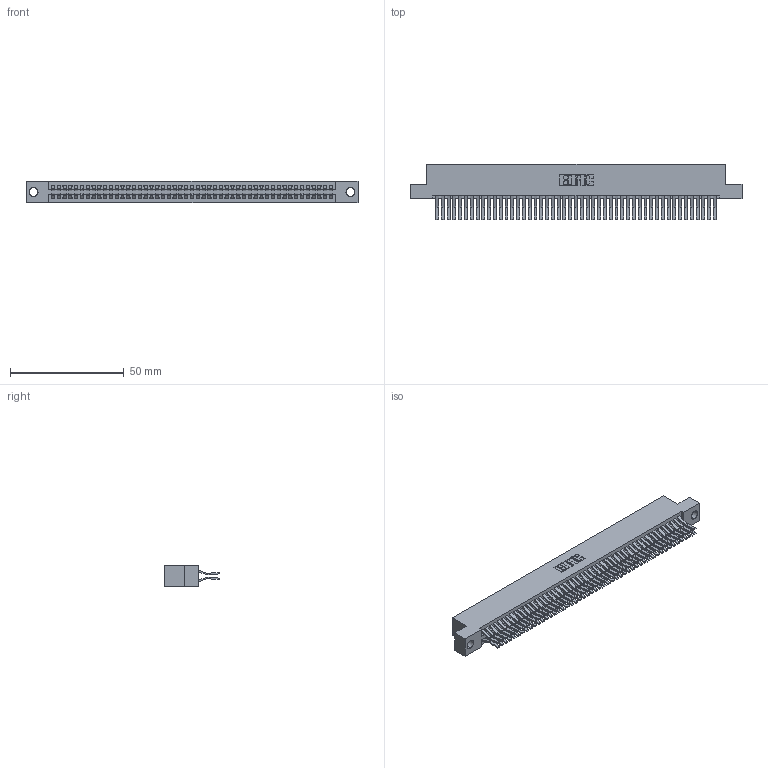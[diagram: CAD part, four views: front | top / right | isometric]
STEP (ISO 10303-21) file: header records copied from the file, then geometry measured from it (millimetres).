
FILE_DESCRIPTION (( 'STEP AP203' ), '1' );
FILE_NAME ('345-098-560-204.STEP', '2021-05-20T18:23:55', ( '' ), ( '' ), 'SwSTEP 2.0', 'SolidWorks 2020', '' );
FILE_SCHEMA (( 'CONFIG_CONTROL_DESIGN' ));
Length unit declared in the file: inch
Products named in the file (3): 345 Part_Flush Mounting Lugs - 0.156 Dia-TI; 345-098-560-204; 345-292-001_560 Tail
Assembly tree (99 placements, depth 2):
  345-098-560-204
    345 Part_Flush Mounting Lugs - 0.156 Dia-TI
    345-292-001_560 Tail  x98
Bounding box: 145.67 x 24.45 x 9.4 mm (x, y, z)
Volume: 14751.8 mm3; surface area: 23444.9 mm2
Topology: 99 solids, 99 shells, 5236 faces, 15567 edges, 10246 vertices
Faces by surface type: plane 3328, cylinder 1908
Entity records: 38011 total; most frequent: CARTESIAN_POINT 6370, ORIENTED_EDGE 6302, DIRECTION 5611, EDGE_CURVE 3151, LINE 2819, VECTOR 2819, VERTEX_POINT 2098, AXIS2_PLACEMENT_3D 1396
